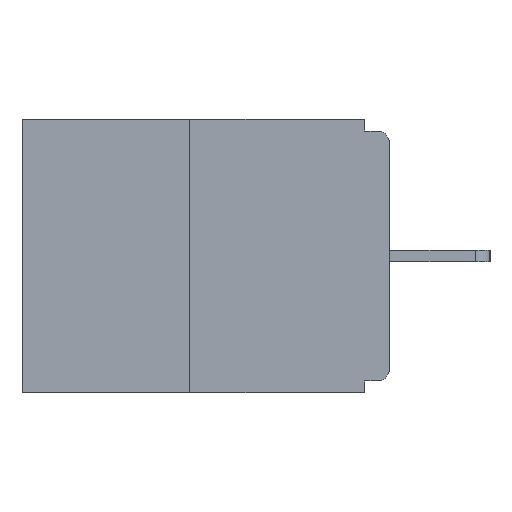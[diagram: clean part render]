
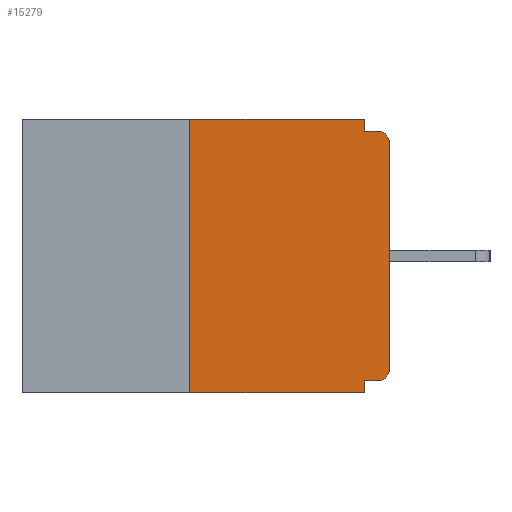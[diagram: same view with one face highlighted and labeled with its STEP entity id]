
A CAD part, left-side view. The second image highlights one B-rep face of the part: STEP entity #15279.
In plain terms, the highlighted planar face has unit normal (-1, 0, 0).
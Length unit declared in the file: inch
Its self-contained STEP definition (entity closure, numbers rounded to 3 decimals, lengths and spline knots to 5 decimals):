
#32 = CARTESIAN_POINT ( 'NONE',  ( 0., 0.031, -0.343 ) ) ;
#377 = ORIENTED_EDGE ( 'NONE', *, *, #2088, .T. ) ;
#880 = CARTESIAN_POINT ( 'NONE',  ( 0., 0.015, -0.328 ) ) ;
#1314 = CARTESIAN_POINT ( 'NONE',  ( 0., 0., -0.313 ) ) ;
#1582 = CARTESIAN_POINT ( 'NONE',  ( 0., 0.031, 0. ) ) ;
#1916 = LINE ( 'NONE', #21613, #21621 ) ;
#2024 = VERTEX_POINT ( 'NONE', #880 ) ;
#2088 = EDGE_CURVE ( 'NONE', #20324, #10917, #12338, .T. ) ;
#2354 = DIRECTION ( 'NONE',  ( 0., 0., -1. ) ) ;
#2363 = EDGE_CURVE ( 'NONE', #2024, #6805, #1916, .T. ) ;
#2553 = EDGE_CURVE ( 'NONE', #19497, #11473, #6705, .T. ) ;
#2669 = ORIENTED_EDGE ( 'NONE', *, *, #2363, .F. ) ;
#2827 = CARTESIAN_POINT ( 'NONE',  ( 0., 0.015, -0.03 ) ) ;
#2943 = LINE ( 'NONE', #10055, #8957 ) ;
#3043 = CARTESIAN_POINT ( 'NONE',  ( 0., 0.031, -0.343 ) ) ;
#4534 = CARTESIAN_POINT ( 'NONE',  ( 0., 0.015, -0.015 ) ) ;
#4891 = AXIS2_PLACEMENT_3D ( 'NONE', #15104, #6390, #13380 ) ;
#4972 = CARTESIAN_POINT ( 'NONE',  ( 0., 0.25, 0. ) ) ;
#5212 = EDGE_CURVE ( 'NONE', #12429, #6761, #10179, .T. ) ;
#6045 = FACE_OUTER_BOUND ( 'NONE', #20534, .T. ) ;
#6261 = ORIENTED_EDGE ( 'NONE', *, *, #17256, .T. ) ;
#6390 = DIRECTION ( 'NONE',  ( 1., 0., 0. ) ) ;
#6705 = LINE ( 'NONE', #4972, #12416 ) ;
#6761 = VERTEX_POINT ( 'NONE', #12810 ) ;
#6805 = VERTEX_POINT ( 'NONE', #16365 ) ;
#6822 = DIRECTION ( 'NONE',  ( 0., 0., -1. ) ) ;
#6825 = LINE ( 'NONE', #6939, #19902 ) ;
#6939 = CARTESIAN_POINT ( 'NONE',  ( 0., 0.46, 0. ) ) ;
#6948 = EDGE_CURVE ( 'NONE', #6805, #8408, #11983, .T. ) ;
#7049 = CARTESIAN_POINT ( 'NONE',  ( 0., 0.031, 0. ) ) ;
#7219 = AXIS2_PLACEMENT_3D ( 'NONE', #2827, #21971, #18766 ) ;
#7544 = ORIENTED_EDGE ( 'NONE', *, *, #20456, .T. ) ;
#7719 = VECTOR ( 'NONE', #17181, 39.37008 ) ;
#7873 = DIRECTION ( 'NONE',  ( 0., 0., 1. ) ) ;
#8091 = PLANE ( 'NONE',  #4891 ) ;
#8231 = EDGE_CURVE ( 'NONE', #11473, #12429, #6825, .T. ) ;
#8408 = VERTEX_POINT ( 'NONE', #32 ) ;
#8715 = VECTOR ( 'NONE', #15655, 39.37008 ) ;
#8957 = VECTOR ( 'NONE', #7873, 39.37008 ) ;
#9164 = DIRECTION ( 'NONE',  ( 0., -1., 0. ) ) ;
#9338 = DIRECTION ( 'NONE',  ( -1., 0., 0. ) ) ;
#10055 = CARTESIAN_POINT ( 'NONE',  ( 0., 0., 0. ) ) ;
#10179 = LINE ( 'NONE', #1582, #7719 ) ;
#10370 = ORIENTED_EDGE ( 'NONE', *, *, #8231, .F. ) ;
#10392 = LINE ( 'NONE', #19208, #8715 ) ;
#10783 = CARTESIAN_POINT ( 'NONE',  ( 0., 0.46, -0.343 ) ) ;
#10917 = VERTEX_POINT ( 'NONE', #4534 ) ;
#11272 = ORIENTED_EDGE ( 'NONE', *, *, #6948, .F. ) ;
#11473 = VERTEX_POINT ( 'NONE', #18497 ) ;
#11983 = LINE ( 'NONE', #3043, #13257 ) ;
#12331 = VERTEX_POINT ( 'NONE', #1314 ) ;
#12338 = CIRCLE ( 'NONE', #7219, 0.015 ) ;
#12416 = VECTOR ( 'NONE', #20568, 39.37008 ) ;
#12429 = VERTEX_POINT ( 'NONE', #7049 ) ;
#12459 = DIRECTION ( 'NONE',  ( 0., 1., 0. ) ) ;
#12596 = ORIENTED_EDGE ( 'NONE', *, *, #5212, .F. ) ;
#12638 = EDGE_CURVE ( 'NONE', #2024, #12331, #15816, .T. ) ;
#12668 = ORIENTED_EDGE ( 'NONE', *, *, #2553, .F. ) ;
#12810 = CARTESIAN_POINT ( 'NONE',  ( 0., 0.031, -0.015 ) ) ;
#12890 = AXIS2_PLACEMENT_3D ( 'NONE', #21483, #9338, #2354 ) ;
#13257 = VECTOR ( 'NONE', #6822, 39.37008 ) ;
#13380 = DIRECTION ( 'NONE',  ( 0., 0., -1. ) ) ;
#13891 = ORIENTED_EDGE ( 'NONE', *, *, #12638, .T. ) ;
#15104 = CARTESIAN_POINT ( 'NONE',  ( 0., 0.46, 0. ) ) ;
#15145 = CARTESIAN_POINT ( 'NONE',  ( 0., 0., -0.03 ) ) ;
#15279 = ADVANCED_FACE ( 'NONE', ( #6045 ), #8091, .F. ) ;
#15655 = DIRECTION ( 'NONE',  ( 0., -1., 0. ) ) ;
#15816 = CIRCLE ( 'NONE', #12890, 0.015 ) ;
#16365 = CARTESIAN_POINT ( 'NONE',  ( 0., 0.031, -0.328 ) ) ;
#16936 = DIRECTION ( 'NONE',  ( 0., -1., 0. ) ) ;
#17181 = DIRECTION ( 'NONE',  ( 0., 0., -1. ) ) ;
#17256 = EDGE_CURVE ( 'NONE', #12331, #20324, #2943, .T. ) ;
#17507 = CARTESIAN_POINT ( 'NONE',  ( 0., 0.25, -0.343 ) ) ;
#18497 = CARTESIAN_POINT ( 'NONE',  ( 0., 0.25, 0. ) ) ;
#18766 = DIRECTION ( 'NONE',  ( 0., 0., -1. ) ) ;
#19208 = CARTESIAN_POINT ( 'NONE',  ( 0., 0., -0.015 ) ) ;
#19296 = VECTOR ( 'NONE', #9164, 39.37008 ) ;
#19497 = VERTEX_POINT ( 'NONE', #17507 ) ;
#19902 = VECTOR ( 'NONE', #16936, 39.37008 ) ;
#20324 = VERTEX_POINT ( 'NONE', #15145 ) ;
#20456 = EDGE_CURVE ( 'NONE', #19497, #8408, #21203, .T. ) ;
#20534 = EDGE_LOOP ( 'NONE', ( #10370, #12668, #7544, #11272, #2669, #13891, #6261, #377, #20761, #12596 ) ) ;
#20568 = DIRECTION ( 'NONE',  ( 0., 0., 1. ) ) ;
#20761 = ORIENTED_EDGE ( 'NONE', *, *, #22306, .F. ) ;
#21203 = LINE ( 'NONE', #10783, #19296 ) ;
#21483 = CARTESIAN_POINT ( 'NONE',  ( 0., 0.015, -0.313 ) ) ;
#21613 = CARTESIAN_POINT ( 'NONE',  ( 0., 0., -0.328 ) ) ;
#21621 = VECTOR ( 'NONE', #12459, 39.37008 ) ;
#21971 = DIRECTION ( 'NONE',  ( -1., 0., 0. ) ) ;
#22306 = EDGE_CURVE ( 'NONE', #6761, #10917, #10392, .T. ) ;
